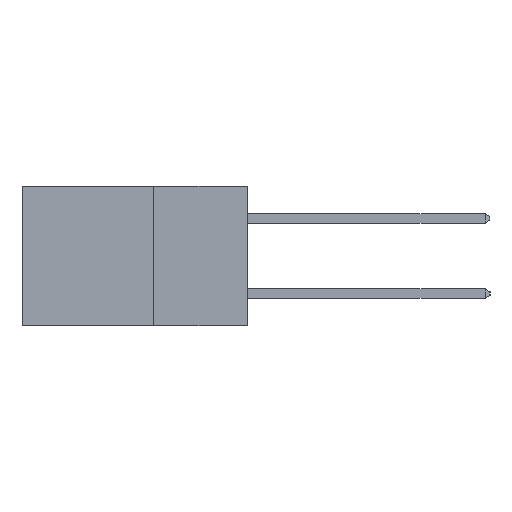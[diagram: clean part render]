
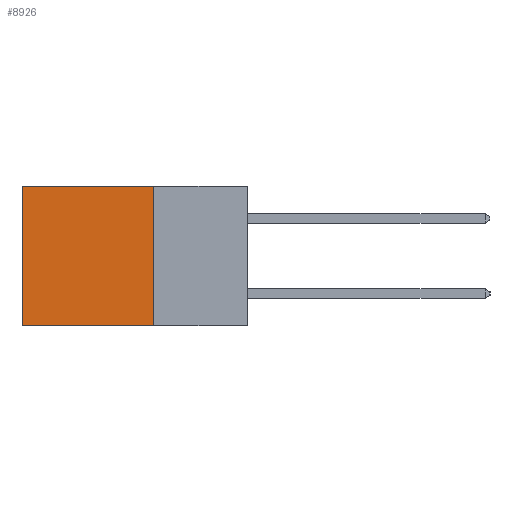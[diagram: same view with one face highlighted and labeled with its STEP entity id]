
A CAD part, left-side view. The second image highlights one B-rep face of the part: STEP entity #8926.
In plain terms, the highlighted planar face has unit normal (-1, 0, 0).
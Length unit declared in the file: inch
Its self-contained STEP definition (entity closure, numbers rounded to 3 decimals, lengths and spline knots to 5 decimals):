
#1281 = EDGE_CURVE ( 'NONE', #3785, #7420, #12792, .T. ) ;
#1285 = CARTESIAN_POINT ( 'NONE',  ( 0.2615, 0.25, -0.37 ) ) ;
#1661 = VECTOR ( 'NONE', #19397, 39.37008 ) ;
#2469 = EDGE_LOOP ( 'NONE', ( #19248, #20376, #11704, #17355 ) ) ;
#2517 = CARTESIAN_POINT ( 'NONE',  ( 0.2615, 0.25, 0. ) ) ;
#2522 = EDGE_CURVE ( 'NONE', #7420, #19069, #6048, .T. ) ;
#2540 = VECTOR ( 'NONE', #12771, 39.37008 ) ;
#2917 = PLANE ( 'NONE',  #14421 ) ;
#3785 = VERTEX_POINT ( 'NONE', #2517 ) ;
#3914 = CARTESIAN_POINT ( 'NONE',  ( 0.2615, 0.25, -0.37 ) ) ;
#4351 = VERTEX_POINT ( 'NONE', #8785 ) ;
#4418 = CARTESIAN_POINT ( 'NONE',  ( 0.2615, 0.6, -0.37 ) ) ;
#4609 = DIRECTION ( 'NONE',  ( 1., 0., 0. ) ) ;
#6048 = LINE ( 'NONE', #7706, #1661 ) ;
#6060 = DIRECTION ( 'NONE',  ( 0., 0., -1. ) ) ;
#7420 = VERTEX_POINT ( 'NONE', #3914 ) ;
#7706 = CARTESIAN_POINT ( 'NONE',  ( 0.2615, 0.25, -0.37 ) ) ;
#8785 = CARTESIAN_POINT ( 'NONE',  ( 0.2615, 0.6, 0. ) ) ;
#8926 = ADVANCED_FACE ( 'NONE', ( #11105 ), #2917, .F. ) ;
#10349 = VECTOR ( 'NONE', #6060, 39.37008 ) ;
#11105 = FACE_OUTER_BOUND ( 'NONE', #2469, .T. ) ;
#11407 = CARTESIAN_POINT ( 'NONE',  ( 0.2615, 0.25, -0.37 ) ) ;
#11459 = DIRECTION ( 'NONE',  ( 0., 0., -1. ) ) ;
#11704 = ORIENTED_EDGE ( 'NONE', *, *, #1281, .F. ) ;
#11829 = LINE ( 'NONE', #20743, #2540 ) ;
#11846 = CARTESIAN_POINT ( 'NONE',  ( 0.2615, 0.6, -0.37 ) ) ;
#12771 = DIRECTION ( 'NONE',  ( 0., 1., 0. ) ) ;
#12792 = LINE ( 'NONE', #11407, #20793 ) ;
#14313 = EDGE_CURVE ( 'NONE', #4351, #19069, #18930, .T. ) ;
#14421 = AXIS2_PLACEMENT_3D ( 'NONE', #1285, #4609, #16015 ) ;
#15602 = EDGE_CURVE ( 'NONE', #3785, #4351, #11829, .T. ) ;
#16015 = DIRECTION ( 'NONE',  ( 0., 0., -1. ) ) ;
#17355 = ORIENTED_EDGE ( 'NONE', *, *, #15602, .T. ) ;
#18930 = LINE ( 'NONE', #4418, #10349 ) ;
#19069 = VERTEX_POINT ( 'NONE', #11846 ) ;
#19248 = ORIENTED_EDGE ( 'NONE', *, *, #14313, .T. ) ;
#19397 = DIRECTION ( 'NONE',  ( 0., 1., 0. ) ) ;
#20376 = ORIENTED_EDGE ( 'NONE', *, *, #2522, .F. ) ;
#20743 = CARTESIAN_POINT ( 'NONE',  ( 0.2615, 0.25, 0. ) ) ;
#20793 = VECTOR ( 'NONE', #11459, 39.37008 ) ;
